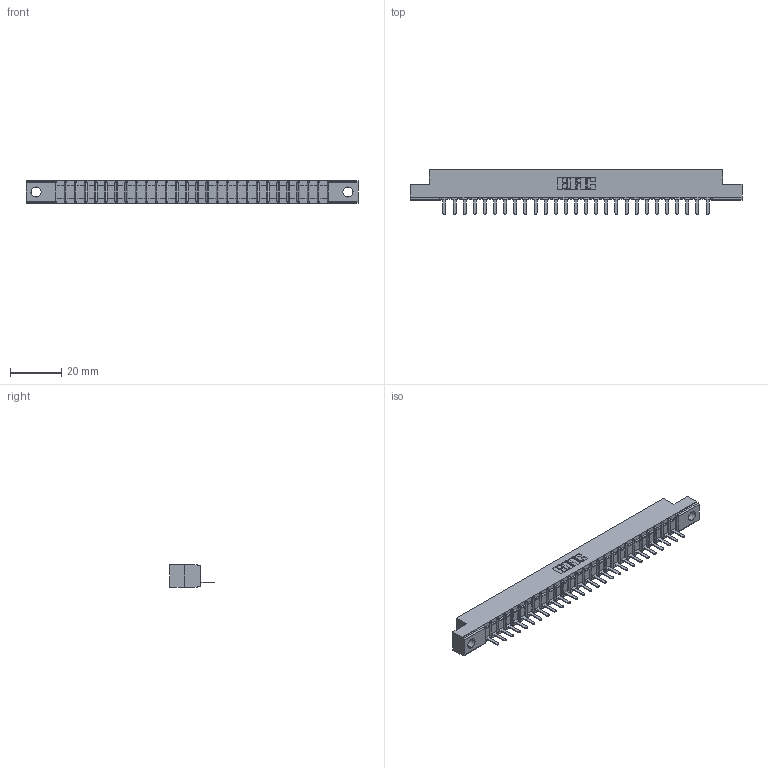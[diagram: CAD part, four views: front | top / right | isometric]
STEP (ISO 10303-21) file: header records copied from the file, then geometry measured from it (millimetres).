
FILE_DESCRIPTION (( 'STEP AP203' ), '1' );
FILE_NAME ('307-027-421-104.STEP', '2020-09-28T05:21:53', ( '' ), ( '' ), 'SwSTEP 2.0', 'SolidWorks 2020', '' );
FILE_SCHEMA (( 'CONFIG_CONTROL_DESIGN' ));
Length unit declared in the file: inch
Products named in the file (3): 307-290-002_521; 307 Part_.156 Dia Mounting Holes; 307-027-421-104
Assembly tree (28 placements, depth 2):
  307-027-421-104
    307 Part_.156 Dia Mounting Holes
    307-290-002_521  x27
Bounding box: 130 x 17.42 x 8.71 mm (x, y, z)
Volume: 8480.4 mm3; surface area: 15609.4 mm2
Topology: 28 solids, 28 shells, 2158 faces, 6623 edges, 4338 vertices
Faces by surface type: plane 1299, cylinder 803, sphere 56
Entity records: 26132 total; most frequent: CARTESIAN_POINT 4410, ORIENTED_EDGE 4398, DIRECTION 4283, EDGE_CURVE 2199, LINE 1685, VECTOR 1685, VERTEX_POINT 1426, AXIS2_PLACEMENT_3D 1299
